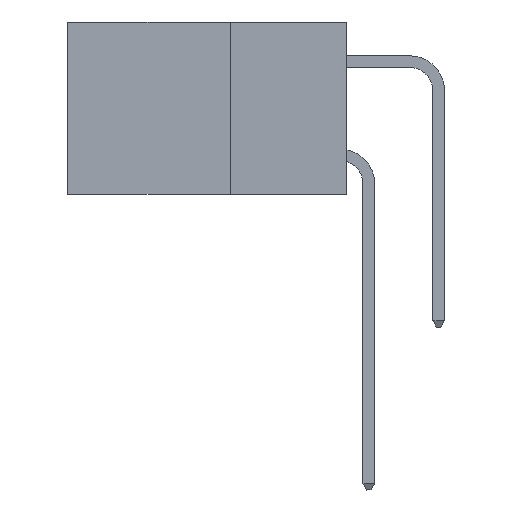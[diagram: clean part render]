
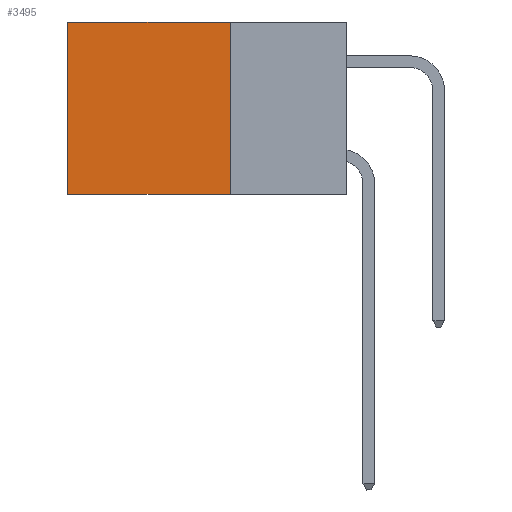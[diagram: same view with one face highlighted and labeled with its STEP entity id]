
A CAD part, left-side view. The second image highlights one B-rep face of the part: STEP entity #3495.
In plain terms, the highlighted planar face has unit normal (-1, 0, 0).
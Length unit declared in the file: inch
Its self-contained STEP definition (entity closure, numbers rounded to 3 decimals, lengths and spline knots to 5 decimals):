
#196 = LINE ( 'NONE', #13609, #2535 ) ;
#990 = ORIENTED_EDGE ( 'NONE', *, *, #4780, .T. ) ;
#1432 = VECTOR ( 'NONE', #6328, 39.37008 ) ;
#1773 = EDGE_CURVE ( 'NONE', #10299, #8346, #8714, .T. ) ;
#2160 = FACE_OUTER_BOUND ( 'NONE', #13490, .T. ) ;
#2379 = ORIENTED_EDGE ( 'NONE', *, *, #2841, .T. ) ;
#2493 = EDGE_CURVE ( 'NONE', #8502, #10299, #196, .T. ) ;
#2535 = VECTOR ( 'NONE', #13124, 39.37008 ) ;
#2841 = EDGE_CURVE ( 'NONE', #8502, #11067, #4304, .T. ) ;
#3495 = ADVANCED_FACE ( 'NONE', ( #2160 ), #7392, .F. ) ;
#4304 = LINE ( 'NONE', #10268, #4663 ) ;
#4663 = VECTOR ( 'NONE', #12313, 39.37008 ) ;
#4780 = EDGE_CURVE ( 'NONE', #11067, #8346, #9998, .T. ) ;
#5152 = ORIENTED_EDGE ( 'NONE', *, *, #1773, .F. ) ;
#6328 = DIRECTION ( 'NONE',  ( 0., 0., -1. ) ) ;
#6349 = CARTESIAN_POINT ( 'NONE',  ( 0.2875, 0.25, 0. ) ) ;
#6466 = DIRECTION ( 'NONE',  ( 0., 0., -1. ) ) ;
#6482 = DIRECTION ( 'NONE',  ( 1., 0., 0. ) ) ;
#6584 = AXIS2_PLACEMENT_3D ( 'NONE', #6349, #6482, #6466 ) ;
#7392 = PLANE ( 'NONE',  #6584 ) ;
#7632 = CARTESIAN_POINT ( 'NONE',  ( 0.2875, 0.6, 0. ) ) ;
#8102 = CARTESIAN_POINT ( 'NONE',  ( 0.2875, 0.6, -0.37 ) ) ;
#8346 = VERTEX_POINT ( 'NONE', #8102 ) ;
#8502 = VERTEX_POINT ( 'NONE', #12726 ) ;
#8714 = LINE ( 'NONE', #9180, #11257 ) ;
#9180 = CARTESIAN_POINT ( 'NONE',  ( 0.2875, 0.25, -0.37 ) ) ;
#9515 = DIRECTION ( 'NONE',  ( 0., 1., 0. ) ) ;
#9998 = LINE ( 'NONE', #7632, #1432 ) ;
#10268 = CARTESIAN_POINT ( 'NONE',  ( 0.2875, 0.25, 0. ) ) ;
#10299 = VERTEX_POINT ( 'NONE', #11333 ) ;
#11067 = VERTEX_POINT ( 'NONE', #13593 ) ;
#11254 = ORIENTED_EDGE ( 'NONE', *, *, #2493, .F. ) ;
#11257 = VECTOR ( 'NONE', #9515, 39.37008 ) ;
#11333 = CARTESIAN_POINT ( 'NONE',  ( 0.2875, 0.25, -0.37 ) ) ;
#12313 = DIRECTION ( 'NONE',  ( 0., 1., 0. ) ) ;
#12726 = CARTESIAN_POINT ( 'NONE',  ( 0.2875, 0.25, 0. ) ) ;
#13124 = DIRECTION ( 'NONE',  ( 0., 0., -1. ) ) ;
#13490 = EDGE_LOOP ( 'NONE', ( #990, #5152, #11254, #2379 ) ) ;
#13593 = CARTESIAN_POINT ( 'NONE',  ( 0.2875, 0.6, 0. ) ) ;
#13609 = CARTESIAN_POINT ( 'NONE',  ( 0.2875, 0.25, 0. ) ) ;
